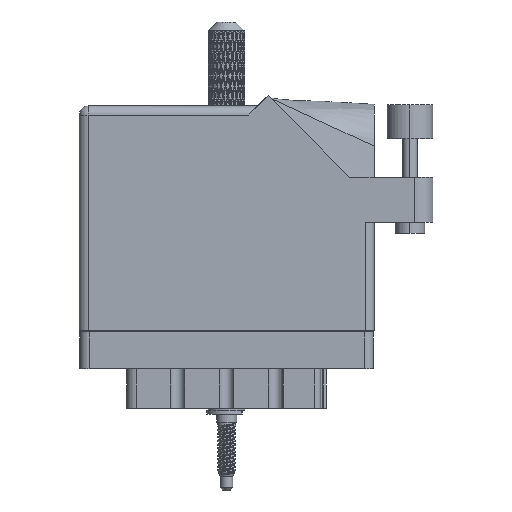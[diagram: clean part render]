
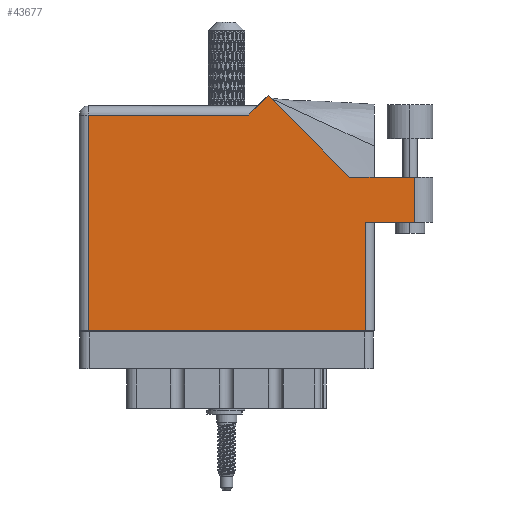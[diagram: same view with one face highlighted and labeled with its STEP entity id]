
A CAD part, front view. The second image highlights one B-rep face of the part: STEP entity #43677.
In plain terms, the highlighted face is planar.
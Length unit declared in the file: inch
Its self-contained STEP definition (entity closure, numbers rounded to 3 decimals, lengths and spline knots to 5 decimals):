
#498 = CARTESIAN_POINT ( 'NONE',  ( 2.285, 1.044, 0. ) ) ;
#997 = DIRECTION ( 'NONE',  ( 0., -1., 0. ) ) ;
#1157 = CARTESIAN_POINT ( 'NONE',  ( 2.41, 1.044, 0. ) ) ;
#2080 = ORIENTED_EDGE ( 'NONE', *, *, #19688, .T. ) ;
#6911 = VERTEX_POINT ( 'NONE', #80475 ) ;
#7861 = VERTEX_POINT ( 'NONE', #94392 ) ;
#8109 = VECTOR ( 'NONE', #20225, 39.37008 ) ;
#8421 = VECTOR ( 'NONE', #82124, 39.37008 ) ;
#9971 = EDGE_LOOP ( 'NONE', ( #48041, #53523, #101653, #65267, #80413, #66198, #72891, #104062, #2080 ) ) ;
#10195 = CARTESIAN_POINT ( 'NONE',  ( 1.948, 0.737, 0. ) ) ;
#12376 = AXIS2_PLACEMENT_3D ( 'NONE', #41474, #16181, #90506 ) ;
#16181 = DIRECTION ( 'NONE',  ( 0., 0., -1. ) ) ;
#19688 = EDGE_CURVE ( 'NONE', #80236, #47789, #82167, .T. ) ;
#20225 = DIRECTION ( 'NONE',  ( 0., 1., 0. ) ) ;
#22768 = EDGE_CURVE ( 'NONE', #102393, #79053, #81518, .T. ) ;
#24406 = CARTESIAN_POINT ( 'NONE',  ( 0., 1.468, 0. ) ) ;
#24866 = PLANE ( 'NONE',  #12376 ) ;
#24933 = DIRECTION ( 'NONE',  ( 1., 0., 0. ) ) ;
#26304 = CARTESIAN_POINT ( 'NONE',  ( 2.01, 0.737, 0. ) ) ;
#30266 = LINE ( 'NONE', #91562, #53530 ) ;
#32861 = CARTESIAN_POINT ( 'NONE',  ( 1.155, 1.468, 0. ) ) ;
#38151 = CARTESIAN_POINT ( 'NONE',  ( 1.948, 0., 0. ) ) ;
#38987 = VECTOR ( 'NONE', #24933, 39.37008 ) ;
#39585 = LINE ( 'NONE', #26304, #42122 ) ;
#39921 = DIRECTION ( 'NONE',  ( 0., 1., 0. ) ) ;
#40325 = EDGE_CURVE ( 'NONE', #6911, #7861, #30266, .T. ) ;
#41474 = CARTESIAN_POINT ( 'NONE',  ( 0., 1.53, 0. ) ) ;
#42122 = VECTOR ( 'NONE', #58762, 39.37008 ) ;
#43071 = FACE_OUTER_BOUND ( 'NONE', #9971, .T. ) ;
#43677 = ADVANCED_FACE ( 'NONE', ( #43071 ), #24866, .F. ) ;
#44926 = LINE ( 'NONE', #1157, #64308 ) ;
#47789 = VERTEX_POINT ( 'NONE', #10195 ) ;
#48041 = ORIENTED_EDGE ( 'NONE', *, *, #94198, .T. ) ;
#49439 = CARTESIAN_POINT ( 'NONE',  ( 2.285, 0.737, 0. ) ) ;
#49982 = VECTOR ( 'NONE', #62173, 39.37008 ) ;
#52473 = CARTESIAN_POINT ( 'NONE',  ( 2.285, 1.044, 0. ) ) ;
#53451 = CARTESIAN_POINT ( 'NONE',  ( 1.28771, 1.60071, 0. ) ) ;
#53523 = ORIENTED_EDGE ( 'NONE', *, *, #80511, .T. ) ;
#53530 = VECTOR ( 'NONE', #997, 39.37008 ) ;
#58762 = DIRECTION ( 'NONE',  ( 1., 0., 0. ) ) ;
#60562 = VERTEX_POINT ( 'NONE', #49439 ) ;
#61085 = CARTESIAN_POINT ( 'NONE',  ( 1.217, 1.53, 0. ) ) ;
#62173 = DIRECTION ( 'NONE',  ( -0.707, -0.707, 0. ) ) ;
#64066 = VECTOR ( 'NONE', #39921, 39.37008 ) ;
#64308 = VECTOR ( 'NONE', #101011, 39.37008 ) ;
#65052 = DIRECTION ( 'NONE',  ( -0.707, 0.707, 0. ) ) ;
#65267 = ORIENTED_EDGE ( 'NONE', *, *, #22768, .T. ) ;
#66119 = CARTESIAN_POINT ( 'NONE',  ( 0., 0., 0. ) ) ;
#66198 = ORIENTED_EDGE ( 'NONE', *, *, #94516, .T. ) ;
#70376 = EDGE_CURVE ( 'NONE', #7861, #80236, #79062, .T. ) ;
#71947 = LINE ( 'NONE', #61085, #49982 ) ;
#72891 = ORIENTED_EDGE ( 'NONE', *, *, #40325, .T. ) ;
#73054 = LINE ( 'NONE', #24406, #8421 ) ;
#75600 = EDGE_CURVE ( 'NONE', #79053, #85249, #71947, .T. ) ;
#76298 = CARTESIAN_POINT ( 'NONE',  ( 1.84442, 1.044, 0. ) ) ;
#79053 = VERTEX_POINT ( 'NONE', #53451 ) ;
#79062 = LINE ( 'NONE', #66119, #38987 ) ;
#80236 = VERTEX_POINT ( 'NONE', #38151 ) ;
#80413 = ORIENTED_EDGE ( 'NONE', *, *, #75600, .T. ) ;
#80475 = CARTESIAN_POINT ( 'NONE',  ( 0.062, 1.468, 0. ) ) ;
#80511 = EDGE_CURVE ( 'NONE', #60562, #104002, #102313, .T. ) ;
#81518 = LINE ( 'NONE', #106133, #89258 ) ;
#82124 = DIRECTION ( 'NONE',  ( -1., 0., 0. ) ) ;
#82167 = LINE ( 'NONE', #89641, #64066 ) ;
#85249 = VERTEX_POINT ( 'NONE', #32861 ) ;
#89258 = VECTOR ( 'NONE', #65052, 39.37008 ) ;
#89641 = CARTESIAN_POINT ( 'NONE',  ( 1.948, 0.737, 0. ) ) ;
#90506 = DIRECTION ( 'NONE',  ( -1., 0., 0. ) ) ;
#91562 = CARTESIAN_POINT ( 'NONE',  ( 0.062, 0., 0. ) ) ;
#92132 = EDGE_CURVE ( 'NONE', #104002, #102393, #44926, .T. ) ;
#94198 = EDGE_CURVE ( 'NONE', #47789, #60562, #39585, .T. ) ;
#94392 = CARTESIAN_POINT ( 'NONE',  ( 0.062, 0., 0. ) ) ;
#94516 = EDGE_CURVE ( 'NONE', #85249, #6911, #73054, .T. ) ;
#101011 = DIRECTION ( 'NONE',  ( -1., 0., 0. ) ) ;
#101653 = ORIENTED_EDGE ( 'NONE', *, *, #92132, .T. ) ;
#102313 = LINE ( 'NONE', #52473, #8109 ) ;
#102393 = VERTEX_POINT ( 'NONE', #76298 ) ;
#104002 = VERTEX_POINT ( 'NONE', #498 ) ;
#104062 = ORIENTED_EDGE ( 'NONE', *, *, #70376, .T. ) ;
#106133 = CARTESIAN_POINT ( 'NONE',  ( 1.84442, 1.044, 0. ) ) ;
